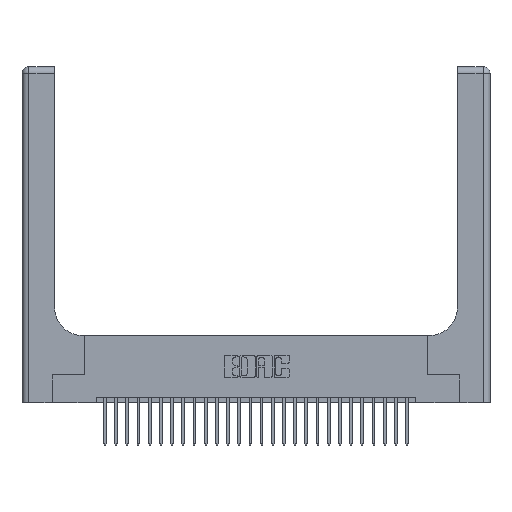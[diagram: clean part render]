
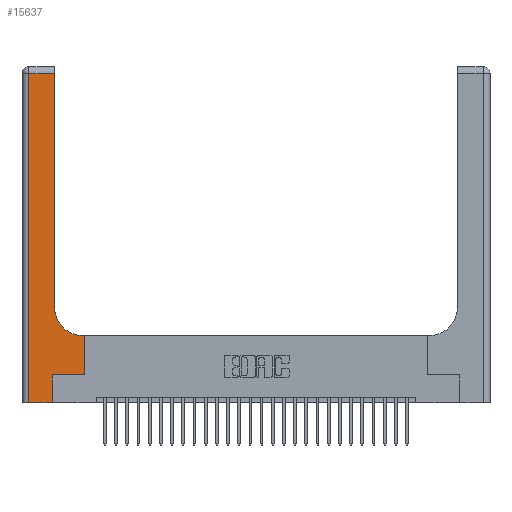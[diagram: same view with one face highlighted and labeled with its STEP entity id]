
A CAD part, top view. The second image highlights one B-rep face of the part: STEP entity #15637.
In plain terms, the highlighted planar face has unit normal (0, 0, 1).
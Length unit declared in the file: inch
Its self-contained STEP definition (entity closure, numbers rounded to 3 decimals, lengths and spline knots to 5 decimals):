
#459 = DIRECTION ( 'NONE',  ( -1., 0., 0. ) ) ;
#1004 = VECTOR ( 'NONE', #21483, 39.37008 ) ;
#1829 = EDGE_CURVE ( 'NONE', #1845, #5480, #13117, .T. ) ;
#1845 = VERTEX_POINT ( 'NONE', #24343 ) ;
#2508 = DIRECTION ( 'NONE',  ( 1., 0., 0. ) ) ;
#2613 = DIRECTION ( 'NONE',  ( -1., 0., 0. ) ) ;
#2630 = ORIENTED_EDGE ( 'NONE', *, *, #4422, .T. ) ;
#2749 = ORIENTED_EDGE ( 'NONE', *, *, #19611, .T. ) ;
#3139 = EDGE_CURVE ( 'NONE', #20087, #20635, #18919, .T. ) ;
#3549 = EDGE_CURVE ( 'NONE', #19144, #6702, #14359, .T. ) ;
#3610 = EDGE_CURVE ( 'NONE', #25354, #26219, #22052, .T. ) ;
#3623 = VECTOR ( 'NONE', #12950, 39.37008 ) ;
#3788 = CARTESIAN_POINT ( 'NONE',  ( 0.06, 3., 0.37 ) ) ;
#4192 = CARTESIAN_POINT ( 'NONE',  ( 0.5585, 0.25, 0.37 ) ) ;
#4422 = EDGE_CURVE ( 'NONE', #6702, #1845, #20591, .T. ) ;
#5120 = EDGE_CURVE ( 'NONE', #20295, #25354, #27972, .T. ) ;
#5418 = ORIENTED_EDGE ( 'NONE', *, *, #3549, .T. ) ;
#5480 = VERTEX_POINT ( 'NONE', #4192 ) ;
#5869 = DIRECTION ( 'NONE',  ( 0., -1., 0. ) ) ;
#6433 = CARTESIAN_POINT ( 'NONE',  ( 0.06, 2.94, 0.37 ) ) ;
#6702 = VERTEX_POINT ( 'NONE', #12894 ) ;
#6814 = DIRECTION ( 'NONE',  ( -1., 0., 0. ) ) ;
#6985 = CARTESIAN_POINT ( 'NONE',  ( 0.2915, 0.6, 0.37 ) ) ;
#7226 = ORIENTED_EDGE ( 'NONE', *, *, #16626, .T. ) ;
#7305 = LINE ( 'NONE', #14501, #21644 ) ;
#7832 = VECTOR ( 'NONE', #2508, 39.37008 ) ;
#10702 = CARTESIAN_POINT ( 'NONE',  ( 0.5585, 0.25, 0.37 ) ) ;
#10820 = ORIENTED_EDGE ( 'NONE', *, *, #1829, .T. ) ;
#11315 = CARTESIAN_POINT ( 'NONE',  ( 0.5415, 0.6, 0.37 ) ) ;
#11330 = ORIENTED_EDGE ( 'NONE', *, *, #3139, .T. ) ;
#11437 = CARTESIAN_POINT ( 'NONE',  ( 0.2915, 2.94, 0.37 ) ) ;
#11654 = DIRECTION ( 'NONE',  ( 0., 0., -1. ) ) ;
#12463 = CARTESIAN_POINT ( 'NONE',  ( 0.06, 0., 0.37 ) ) ;
#12683 = VECTOR ( 'NONE', #6814, 39.37008 ) ;
#12894 = CARTESIAN_POINT ( 'NONE',  ( 0.269, 0., 0.37 ) ) ;
#12950 = DIRECTION ( 'NONE',  ( 0., 1., 0. ) ) ;
#13116 = LINE ( 'NONE', #10702, #3623 ) ;
#13117 = LINE ( 'NONE', #22580, #7832 ) ;
#14359 = LINE ( 'NONE', #24059, #1004 ) ;
#14389 = DIRECTION ( 'NONE',  ( 0., 1., 0. ) ) ;
#14501 = CARTESIAN_POINT ( 'NONE',  ( 0.2915, 3., 0.37 ) ) ;
#14879 = DIRECTION ( 'NONE',  ( 0., 1., 0. ) ) ;
#15637 = ADVANCED_FACE ( 'NONE', ( #24013 ), #18364, .F. ) ;
#16461 = AXIS2_PLACEMENT_3D ( 'NONE', #24261, #22163, #24453 ) ;
#16626 = EDGE_CURVE ( 'NONE', #5480, #20295, #13116, .T. ) ;
#16885 = CARTESIAN_POINT ( 'NONE',  ( 0.5585, 0.6, 0.37 ) ) ;
#17715 = EDGE_LOOP ( 'NONE', ( #2749, #11330, #25453, #5418, #2630, #10820, #7226, #24742, #23308 ) ) ;
#18364 = PLANE ( 'NONE',  #23864 ) ;
#18919 = LINE ( 'NONE', #24647, #12683 ) ;
#19144 = VERTEX_POINT ( 'NONE', #12463 ) ;
#19207 = EDGE_CURVE ( 'NONE', #20635, #19144, #21321, .T. ) ;
#19545 = VECTOR ( 'NONE', #14879, 39.37008 ) ;
#19611 = EDGE_CURVE ( 'NONE', #26219, #20087, #7305, .T. ) ;
#20087 = VERTEX_POINT ( 'NONE', #11437 ) ;
#20295 = VERTEX_POINT ( 'NONE', #16885 ) ;
#20591 = LINE ( 'NONE', #28321, #19545 ) ;
#20635 = VERTEX_POINT ( 'NONE', #6433 ) ;
#21321 = LINE ( 'NONE', #3788, #23439 ) ;
#21483 = DIRECTION ( 'NONE',  ( 1., 0., 0. ) ) ;
#21644 = VECTOR ( 'NONE', #14389, 39.37008 ) ;
#21973 = VECTOR ( 'NONE', #459, 39.37008 ) ;
#22052 = CIRCLE ( 'NONE', #16461, 0.25 ) ;
#22163 = DIRECTION ( 'NONE',  ( 0., 0., -1. ) ) ;
#22580 = CARTESIAN_POINT ( 'NONE',  ( 0.269, 0.25, 0.37 ) ) ;
#22989 = CARTESIAN_POINT ( 'NONE',  ( 0., 3., 0.37 ) ) ;
#23308 = ORIENTED_EDGE ( 'NONE', *, *, #3610, .T. ) ;
#23401 = CARTESIAN_POINT ( 'NONE',  ( 0.2915, 0.85, 0.37 ) ) ;
#23439 = VECTOR ( 'NONE', #5869, 39.37008 ) ;
#23864 = AXIS2_PLACEMENT_3D ( 'NONE', #22989, #11654, #2613 ) ;
#24013 = FACE_OUTER_BOUND ( 'NONE', #17715, .T. ) ;
#24059 = CARTESIAN_POINT ( 'NONE',  ( 0., 0., 0.37 ) ) ;
#24261 = CARTESIAN_POINT ( 'NONE',  ( 0.5415, 0.85, 0.37 ) ) ;
#24343 = CARTESIAN_POINT ( 'NONE',  ( 0.269, 0.25, 0.37 ) ) ;
#24453 = DIRECTION ( 'NONE',  ( 1., 0., 0. ) ) ;
#24647 = CARTESIAN_POINT ( 'NONE',  ( 0., 2.94, 0.37 ) ) ;
#24742 = ORIENTED_EDGE ( 'NONE', *, *, #5120, .T. ) ;
#25354 = VERTEX_POINT ( 'NONE', #11315 ) ;
#25453 = ORIENTED_EDGE ( 'NONE', *, *, #19207, .T. ) ;
#26219 = VERTEX_POINT ( 'NONE', #23401 ) ;
#27972 = LINE ( 'NONE', #6985, #21973 ) ;
#28321 = CARTESIAN_POINT ( 'NONE',  ( 0.269, 0., 0.37 ) ) ;
